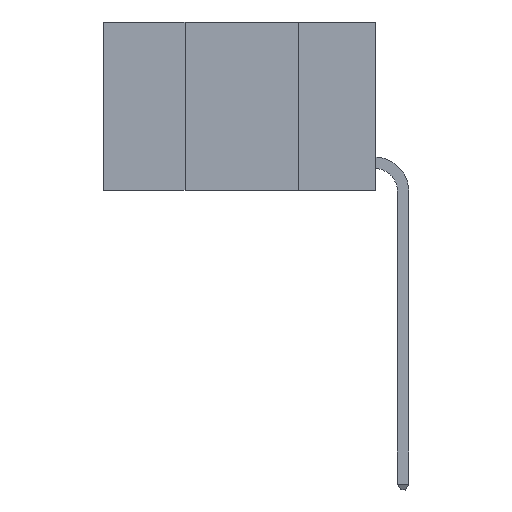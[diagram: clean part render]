
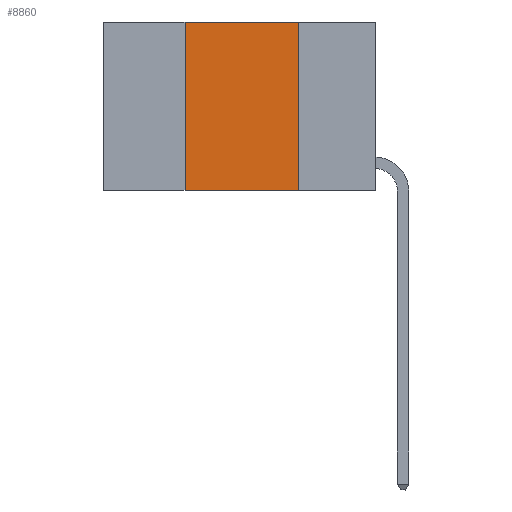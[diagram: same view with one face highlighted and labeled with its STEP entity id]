
A CAD part, left-side view. The second image highlights one B-rep face of the part: STEP entity #8860.
In plain terms, the highlighted planar face has unit normal (-1, 0, 0).
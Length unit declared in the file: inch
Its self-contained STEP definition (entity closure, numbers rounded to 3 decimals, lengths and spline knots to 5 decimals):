
#557 = VECTOR ( 'NONE', #15943, 39.37008 ) ;
#2024 = CARTESIAN_POINT ( 'NONE',  ( 0., 0.42, 0. ) ) ;
#2038 = VERTEX_POINT ( 'NONE', #9625 ) ;
#2180 = ORIENTED_EDGE ( 'NONE', *, *, #6694, .F. ) ;
#2564 = VECTOR ( 'NONE', #3438, 39.37008 ) ;
#2601 = EDGE_CURVE ( 'NONE', #3221, #3991, #6221, .T. ) ;
#2871 = DIRECTION ( 'NONE',  ( 0., -1., 0. ) ) ;
#2897 = AXIS2_PLACEMENT_3D ( 'NONE', #15730, #11809, #3725 ) ;
#2991 = VECTOR ( 'NONE', #2871, 39.37008 ) ;
#3221 = VERTEX_POINT ( 'NONE', #6902 ) ;
#3333 = CARTESIAN_POINT ( 'NONE',  ( 0., 0.6, 0. ) ) ;
#3438 = DIRECTION ( 'NONE',  ( 0., 0., 1. ) ) ;
#3565 = EDGE_CURVE ( 'NONE', #2038, #13705, #11647, .T. ) ;
#3716 = DIRECTION ( 'NONE',  ( 0., -1., 0. ) ) ;
#3725 = DIRECTION ( 'NONE',  ( 0., 0., -1. ) ) ;
#3991 = VERTEX_POINT ( 'NONE', #9909 ) ;
#5126 = FACE_OUTER_BOUND ( 'NONE', #9638, .T. ) ;
#5598 = ORIENTED_EDGE ( 'NONE', *, *, #12781, .F. ) ;
#6221 = LINE ( 'NONE', #3333, #2991 ) ;
#6625 = CARTESIAN_POINT ( 'NONE',  ( 0., 0.17, 0. ) ) ;
#6694 = EDGE_CURVE ( 'NONE', #3991, #13705, #11465, .T. ) ;
#6902 = CARTESIAN_POINT ( 'NONE',  ( 0., 0.42, 0. ) ) ;
#7950 = CARTESIAN_POINT ( 'NONE',  ( 0., 0.17, -0.37 ) ) ;
#8860 = ADVANCED_FACE ( 'NONE', ( #5126 ), #13073, .F. ) ;
#9607 = ORIENTED_EDGE ( 'NONE', *, *, #2601, .F. ) ;
#9625 = CARTESIAN_POINT ( 'NONE',  ( 0., 0.42, -0.37 ) ) ;
#9638 = EDGE_LOOP ( 'NONE', ( #2180, #9607, #5598, #12296 ) ) ;
#9909 = CARTESIAN_POINT ( 'NONE',  ( 0., 0.17, 0. ) ) ;
#10459 = CARTESIAN_POINT ( 'NONE',  ( 0., 0.6, -0.37 ) ) ;
#11225 = VECTOR ( 'NONE', #3716, 39.37008 ) ;
#11465 = LINE ( 'NONE', #6625, #557 ) ;
#11647 = LINE ( 'NONE', #10459, #11225 ) ;
#11809 = DIRECTION ( 'NONE',  ( 1., 0., 0. ) ) ;
#12296 = ORIENTED_EDGE ( 'NONE', *, *, #3565, .T. ) ;
#12781 = EDGE_CURVE ( 'NONE', #2038, #3221, #14553, .T. ) ;
#13073 = PLANE ( 'NONE',  #2897 ) ;
#13705 = VERTEX_POINT ( 'NONE', #7950 ) ;
#14553 = LINE ( 'NONE', #2024, #2564 ) ;
#15730 = CARTESIAN_POINT ( 'NONE',  ( 0., 0.6, 0. ) ) ;
#15943 = DIRECTION ( 'NONE',  ( 0., 0., -1. ) ) ;
